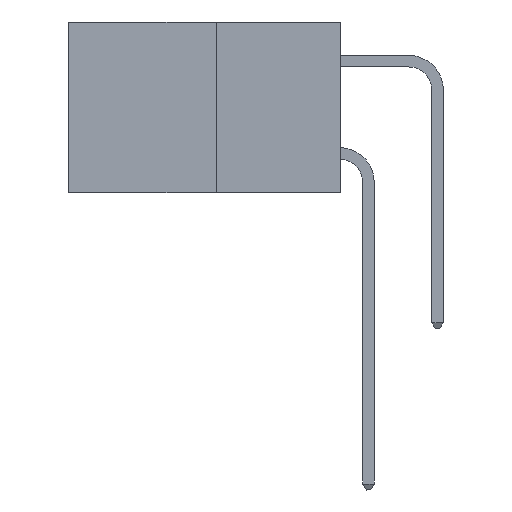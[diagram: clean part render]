
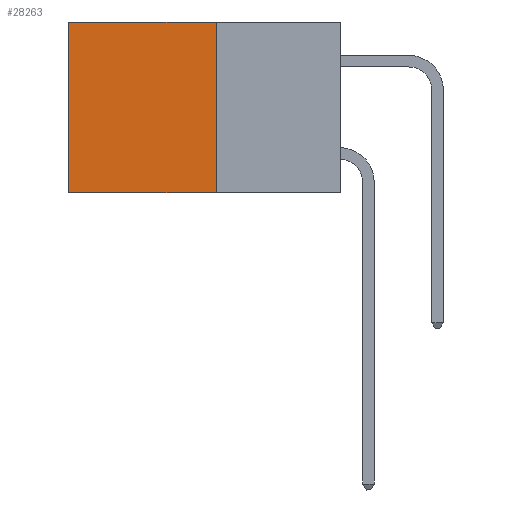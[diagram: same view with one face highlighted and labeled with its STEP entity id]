
A CAD part, left-side view. The second image highlights one B-rep face of the part: STEP entity #28263.
In plain terms, the highlighted planar face has unit normal (-1, 0, 0).
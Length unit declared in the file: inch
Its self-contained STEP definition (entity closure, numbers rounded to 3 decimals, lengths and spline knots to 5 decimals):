
#138 = PLANE ( 'NONE',  #26249 ) ;
#364 = EDGE_CURVE ( 'NONE', #17788, #13910, #25716, .T. ) ;
#1652 = VECTOR ( 'NONE', #17492, 39.37008 ) ;
#2259 = EDGE_CURVE ( 'NONE', #25427, #26561, #13923, .T. ) ;
#2451 = DIRECTION ( 'NONE',  ( 0., 0., -1. ) ) ;
#2948 = DIRECTION ( 'NONE',  ( 0., 1., 0. ) ) ;
#4413 = VECTOR ( 'NONE', #2948, 39.37008 ) ;
#5400 = EDGE_LOOP ( 'NONE', ( #19392, #16640, #21553, #25491 ) ) ;
#10620 = LINE ( 'NONE', #12179, #4413 ) ;
#11726 = DIRECTION ( 'NONE',  ( 0., 1., 0. ) ) ;
#12179 = CARTESIAN_POINT ( 'NONE',  ( 0.277, 0.27, -0.37 ) ) ;
#13248 = VECTOR ( 'NONE', #18862, 39.37008 ) ;
#13784 = CARTESIAN_POINT ( 'NONE',  ( 0.277, 0.27, -0.37 ) ) ;
#13910 = VERTEX_POINT ( 'NONE', #25360 ) ;
#13923 = LINE ( 'NONE', #13784, #13248 ) ;
#14641 = EDGE_CURVE ( 'NONE', #25427, #17788, #23323, .T. ) ;
#16121 = DIRECTION ( 'NONE',  ( 1., 0., 0. ) ) ;
#16586 = CARTESIAN_POINT ( 'NONE',  ( 0.277, 0.59, 0. ) ) ;
#16640 = ORIENTED_EDGE ( 'NONE', *, *, #17786, .F. ) ;
#16902 = CARTESIAN_POINT ( 'NONE',  ( 0.277, 0.59, -0.37 ) ) ;
#17367 = VECTOR ( 'NONE', #11726, 39.37008 ) ;
#17492 = DIRECTION ( 'NONE',  ( 0., 0., -1. ) ) ;
#17786 = EDGE_CURVE ( 'NONE', #26561, #13910, #10620, .T. ) ;
#17788 = VERTEX_POINT ( 'NONE', #16586 ) ;
#18862 = DIRECTION ( 'NONE',  ( 0., 0., -1. ) ) ;
#19392 = ORIENTED_EDGE ( 'NONE', *, *, #364, .T. ) ;
#21363 = CARTESIAN_POINT ( 'NONE',  ( 0.277, 0.27, -0.37 ) ) ;
#21553 = ORIENTED_EDGE ( 'NONE', *, *, #2259, .F. ) ;
#22751 = CARTESIAN_POINT ( 'NONE',  ( 0.277, 0.27, -0.37 ) ) ;
#23323 = LINE ( 'NONE', #27265, #17367 ) ;
#23763 = FACE_OUTER_BOUND ( 'NONE', #5400, .T. ) ;
#25360 = CARTESIAN_POINT ( 'NONE',  ( 0.277, 0.59, -0.37 ) ) ;
#25427 = VERTEX_POINT ( 'NONE', #27429 ) ;
#25491 = ORIENTED_EDGE ( 'NONE', *, *, #14641, .T. ) ;
#25716 = LINE ( 'NONE', #16902, #1652 ) ;
#26249 = AXIS2_PLACEMENT_3D ( 'NONE', #22751, #16121, #2451 ) ;
#26561 = VERTEX_POINT ( 'NONE', #21363 ) ;
#27265 = CARTESIAN_POINT ( 'NONE',  ( 0.277, 0.27, 0. ) ) ;
#27429 = CARTESIAN_POINT ( 'NONE',  ( 0.277, 0.27, 0. ) ) ;
#28263 = ADVANCED_FACE ( 'NONE', ( #23763 ), #138, .F. ) ;
